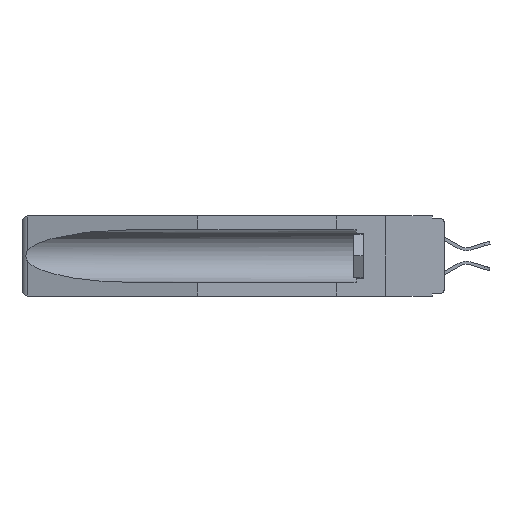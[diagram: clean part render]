
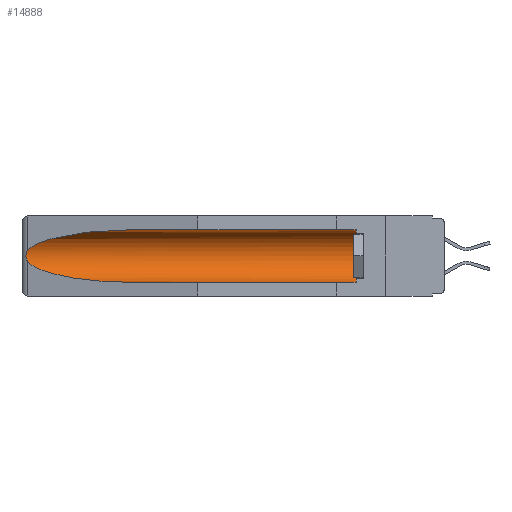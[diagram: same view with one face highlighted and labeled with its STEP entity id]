
A CAD part, left-side view. The second image highlights one B-rep face of the part: STEP entity #14888.
In plain terms, the highlighted cylindrical face has radius 2.857 mm (diameter 5.715 mm), a partial arc.
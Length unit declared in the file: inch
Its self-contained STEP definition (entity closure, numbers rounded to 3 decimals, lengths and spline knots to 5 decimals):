
#14 = CARTESIAN_POINT ( 'NONE',  ( 0.21114, 1.30732, -0.284 ) ) ;
#97 = DIRECTION ( 'NONE',  ( 0., 1., 0. ) ) ;
#162 = VERTEX_POINT ( 'NONE', #14613 ) ;
#998 = CARTESIAN_POINT ( 'NONE',  ( 0.2673, 1.53269, -0.17917 ) ) ;
#1038 =( BOUNDED_CURVE ( )  B_SPLINE_CURVE ( 3, ( #17408, #3770, #10441, #9660 ),
 .UNSPECIFIED., .F., .T. ) 
 B_SPLINE_CURVE_WITH_KNOTS ( ( 4, 4 ),
 ( 4.71239, 6.08839 ),
 .UNSPECIFIED. ) 
 CURVE ( )  GEOMETRIC_REPRESENTATION_ITEM ( )  RATIONAL_B_SPLINE_CURVE ( ( 1., 0.848, 0.848, 1. ) ) 
 REPRESENTATION_ITEM ( '' )  );
#1069 = CARTESIAN_POINT ( 'NONE',  ( 0.26537, 1.52718, -0.19328 ) ) ;
#1158 = EDGE_CURVE ( 'NONE', #8243, #12159, #1038, .T. ) ;
#1218 = CARTESIAN_POINT ( 'NONE',  ( 0.2675, 1.53308, -0.16763 ) ) ;
#1376 = CARTESIAN_POINT ( 'NONE',  ( 0.155, -0.30754, -0.059 ) ) ;
#1680 = CARTESIAN_POINT ( 'NONE',  ( 0.155, 0.126, -0.284 ) ) ;
#2509 = ORIENTED_EDGE ( 'NONE', *, *, #11424, .T. ) ;
#2573 = DIRECTION ( 'NONE',  ( 0., 0., 1. ) ) ;
#3332 = ORIENTED_EDGE ( 'NONE', *, *, #16363, .T. ) ;
#3548 = CARTESIAN_POINT ( 'NONE',  ( 0.155, -0.30754, -0.284 ) ) ;
#3770 = CARTESIAN_POINT ( 'NONE',  ( 0.21114, 1.30732, -0.059 ) ) ;
#3779 =( BOUNDED_CURVE ( )  B_SPLINE_CURVE ( 3, ( #9912, #9981, #14, #8115 ),
 .UNSPECIFIED., .F., .F. ) 
 B_SPLINE_CURVE_WITH_KNOTS ( ( 4, 4 ),
 ( 0.1948, 1.5708 ),
 .UNSPECIFIED. ) 
 CURVE ( )  GEOMETRIC_REPRESENTATION_ITEM ( )  RATIONAL_B_SPLINE_CURVE ( ( 1., 0.848, 0.848, 1. ) ) 
 REPRESENTATION_ITEM ( '' )  );
#4799 = VECTOR ( 'NONE', #14864, 39.37008 ) ;
#4996 = VERTEX_POINT ( 'NONE', #19510 ) ;
#5224 = LINE ( 'NONE', #3548, #7034 ) ;
#6039 = B_SPLINE_CURVE_WITH_KNOTS ( 'NONE', 3,
 ( #17933, #11116, #20984, #10977, #1218, #14370, #998, #21057, #7703, #1069 ),
 .UNSPECIFIED., .F., .F.,
 ( 4, 2, 2, 2, 4 ),
 ( 0., 0.00029, 0.00058, 0.00087, 0.00117 ),
 .UNSPECIFIED. ) ;
#6352 = CARTESIAN_POINT ( 'NONE',  ( 0.26537, 1.52718, -0.14972 ) ) ;
#7034 = VECTOR ( 'NONE', #97, 39.37008 ) ;
#7703 = CARTESIAN_POINT ( 'NONE',  ( 0.26597, 1.5296, -0.19026 ) ) ;
#7919 = CARTESIAN_POINT ( 'NONE',  ( 0.155, 1.07973, -0.059 ) ) ;
#7970 = CARTESIAN_POINT ( 'NONE',  ( 0.26537, 1.52718, -0.19328 ) ) ;
#8115 = CARTESIAN_POINT ( 'NONE',  ( 0.155, 1.07973, -0.284 ) ) ;
#8205 = EDGE_LOOP ( 'NONE', ( #16069, #3332, #18783, #17572, #2509, #21334 ) ) ;
#8243 = VERTEX_POINT ( 'NONE', #7919 ) ;
#8486 = EDGE_CURVE ( 'NONE', #20342, #162, #5224, .T. ) ;
#9238 = LINE ( 'NONE', #1376, #4799 ) ;
#9660 = CARTESIAN_POINT ( 'NONE',  ( 0.26537, 1.52718, -0.14972 ) ) ;
#9912 = CARTESIAN_POINT ( 'NONE',  ( 0.26537, 1.52718, -0.19328 ) ) ;
#9981 = CARTESIAN_POINT ( 'NONE',  ( 0.25451, 1.48313, -0.24835 ) ) ;
#10441 = CARTESIAN_POINT ( 'NONE',  ( 0.25451, 1.48313, -0.09465 ) ) ;
#10977 = CARTESIAN_POINT ( 'NONE',  ( 0.2673, 1.5327, -0.16383 ) ) ;
#11116 = CARTESIAN_POINT ( 'NONE',  ( 0.26597, 1.52961, -0.15275 ) ) ;
#11424 = EDGE_CURVE ( 'NONE', #20342, #4996, #15729, .T. ) ;
#11951 = VERTEX_POINT ( 'NONE', #7970 ) ;
#12159 = VERTEX_POINT ( 'NONE', #6352 ) ;
#12460 = DIRECTION ( 'NONE',  ( 0., -1., 0. ) ) ;
#12495 = CARTESIAN_POINT ( 'NONE',  ( 0.155, -0.30754, -0.1715 ) ) ;
#13281 = FACE_OUTER_BOUND ( 'NONE', #8205, .T. ) ;
#14167 = DIRECTION ( 'NONE',  ( 0., 1., 0. ) ) ;
#14370 = CARTESIAN_POINT ( 'NONE',  ( 0.2675, 1.53308, -0.17534 ) ) ;
#14613 = CARTESIAN_POINT ( 'NONE',  ( 0.155, 1.07973, -0.284 ) ) ;
#14864 = DIRECTION ( 'NONE',  ( 0., 1., 0. ) ) ;
#14888 = ADVANCED_FACE ( 'NONE', ( #13281 ), #18307, .F. ) ;
#15664 = CARTESIAN_POINT ( 'NONE',  ( 0.155, 0.126, -0.1715 ) ) ;
#15729 = CIRCLE ( 'NONE', #17753, 0.1125 ) ;
#16069 = ORIENTED_EDGE ( 'NONE', *, *, #1158, .T. ) ;
#16363 = EDGE_CURVE ( 'NONE', #12159, #11951, #6039, .T. ) ;
#17163 = EDGE_CURVE ( 'NONE', #11951, #162, #3779, .T. ) ;
#17408 = CARTESIAN_POINT ( 'NONE',  ( 0.155, 1.07973, -0.059 ) ) ;
#17572 = ORIENTED_EDGE ( 'NONE', *, *, #8486, .F. ) ;
#17753 = AXIS2_PLACEMENT_3D ( 'NONE', #15664, #12460, #2573 ) ;
#17933 = CARTESIAN_POINT ( 'NONE',  ( 0.26537, 1.52718, -0.14972 ) ) ;
#18223 = AXIS2_PLACEMENT_3D ( 'NONE', #12495, #14167, #18966 ) ;
#18307 = CYLINDRICAL_SURFACE ( 'NONE', #18223, 0.1125 ) ;
#18783 = ORIENTED_EDGE ( 'NONE', *, *, #17163, .T. ) ;
#18933 = EDGE_CURVE ( 'NONE', #4996, #8243, #9238, .T. ) ;
#18966 = DIRECTION ( 'NONE',  ( 0., 0., 1. ) ) ;
#19510 = CARTESIAN_POINT ( 'NONE',  ( 0.155, 0.126, -0.059 ) ) ;
#20342 = VERTEX_POINT ( 'NONE', #1680 ) ;
#20984 = CARTESIAN_POINT ( 'NONE',  ( 0.26654, 1.53092, -0.15636 ) ) ;
#21057 = CARTESIAN_POINT ( 'NONE',  ( 0.26655, 1.53094, -0.18657 ) ) ;
#21334 = ORIENTED_EDGE ( 'NONE', *, *, #18933, .T. ) ;
